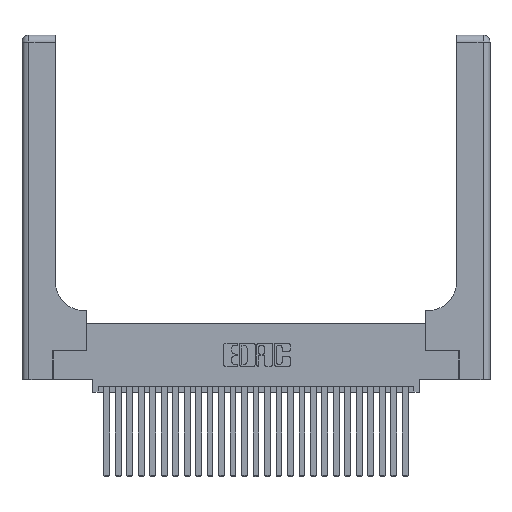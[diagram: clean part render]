
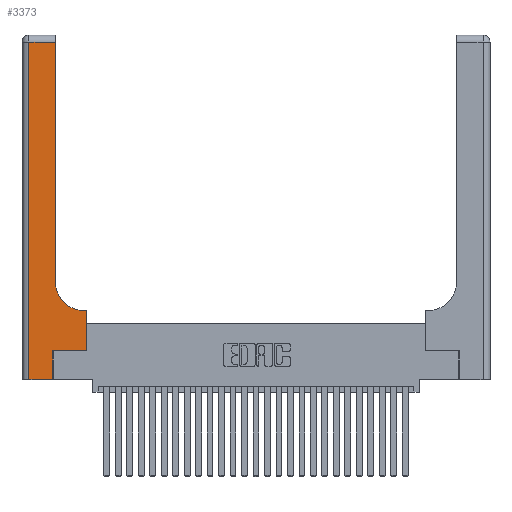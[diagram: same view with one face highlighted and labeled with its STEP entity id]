
A CAD part, top view. The second image highlights one B-rep face of the part: STEP entity #3373.
In plain terms, the highlighted planar face has unit normal (0, 0, 1).
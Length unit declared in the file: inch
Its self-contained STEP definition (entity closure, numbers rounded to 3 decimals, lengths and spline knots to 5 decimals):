
#2364 = CARTESIAN_POINT ( 'NONE',  ( 0.269, 0., 0.37 ) ) ;
#2859 = CARTESIAN_POINT ( 'NONE',  ( 0.2915, 3., 0.37 ) ) ;
#2923 = CARTESIAN_POINT ( 'NONE',  ( 0.2915, 2.94, 0.37 ) ) ;
#2935 = EDGE_CURVE ( 'NONE', #10302, #12934, #21000, .T. ) ;
#3134 = LINE ( 'NONE', #16688, #11346 ) ;
#3373 = ADVANCED_FACE ( 'NONE', ( #4722 ), #11329, .F. ) ;
#3990 = CARTESIAN_POINT ( 'NONE',  ( 0.269, 0.25, 0.37 ) ) ;
#4154 = ORIENTED_EDGE ( 'NONE', *, *, #14127, .T. ) ;
#4536 = DIRECTION ( 'NONE',  ( 0., 1., 0. ) ) ;
#4601 = ORIENTED_EDGE ( 'NONE', *, *, #17300, .T. ) ;
#4671 = CARTESIAN_POINT ( 'NONE',  ( 0.06, 3., 0.37 ) ) ;
#4722 = FACE_OUTER_BOUND ( 'NONE', #21635, .T. ) ;
#4834 = CARTESIAN_POINT ( 'NONE',  ( 0.269, 0.25, 0.37 ) ) ;
#4879 = CARTESIAN_POINT ( 'NONE',  ( 0., 3., 0.37 ) ) ;
#4957 = DIRECTION ( 'NONE',  ( 1., 0., 0. ) ) ;
#5031 = DIRECTION ( 'NONE',  ( 0., 1., 0. ) ) ;
#5175 = DIRECTION ( 'NONE',  ( 0., 1., 0. ) ) ;
#5514 = VECTOR ( 'NONE', #4957, 39.37008 ) ;
#5590 = VECTOR ( 'NONE', #5175, 39.37008 ) ;
#5608 = CIRCLE ( 'NONE', #23558, 0.25 ) ;
#6790 = DIRECTION ( 'NONE',  ( 0., -1., 0. ) ) ;
#6842 = CARTESIAN_POINT ( 'NONE',  ( 0.269, 0., 0.37 ) ) ;
#6924 = VERTEX_POINT ( 'NONE', #21004 ) ;
#7372 = CARTESIAN_POINT ( 'NONE',  ( 0.06, 2.94, 0.37 ) ) ;
#7584 = VERTEX_POINT ( 'NONE', #26493 ) ;
#8196 = VERTEX_POINT ( 'NONE', #23584 ) ;
#8444 = EDGE_CURVE ( 'NONE', #8196, #7584, #10663, .T. ) ;
#8859 = VECTOR ( 'NONE', #5031, 39.37008 ) ;
#8915 = ORIENTED_EDGE ( 'NONE', *, *, #8444, .T. ) ;
#9734 = EDGE_CURVE ( 'NONE', #12934, #21002, #12864, .T. ) ;
#10302 = VERTEX_POINT ( 'NONE', #7372 ) ;
#10546 = DIRECTION ( 'NONE',  ( -1., 0., 0. ) ) ;
#10648 = ORIENTED_EDGE ( 'NONE', *, *, #25148, .T. ) ;
#10663 = LINE ( 'NONE', #16433, #12419 ) ;
#11214 = VERTEX_POINT ( 'NONE', #3990 ) ;
#11329 = PLANE ( 'NONE',  #25306 ) ;
#11346 = VECTOR ( 'NONE', #10546, 39.37008 ) ;
#12419 = VECTOR ( 'NONE', #16619, 39.37008 ) ;
#12864 = LINE ( 'NONE', #22420, #5514 ) ;
#12934 = VERTEX_POINT ( 'NONE', #14301 ) ;
#14127 = EDGE_CURVE ( 'NONE', #6924, #8196, #26868, .T. ) ;
#14301 = CARTESIAN_POINT ( 'NONE',  ( 0.06, 0., 0.37 ) ) ;
#15295 = EDGE_CURVE ( 'NONE', #21002, #11214, #24083, .T. ) ;
#16262 = VERTEX_POINT ( 'NONE', #2923 ) ;
#16278 = VECTOR ( 'NONE', #20381, 39.37008 ) ;
#16433 = CARTESIAN_POINT ( 'NONE',  ( 0.2915, 0.6, 0.37 ) ) ;
#16619 = DIRECTION ( 'NONE',  ( -1., 0., 0. ) ) ;
#16688 = CARTESIAN_POINT ( 'NONE',  ( 0., 2.94, 0.37 ) ) ;
#16888 = CARTESIAN_POINT ( 'NONE',  ( 0.2915, 0.85, 0.37 ) ) ;
#17300 = EDGE_CURVE ( 'NONE', #21382, #16262, #20516, .T. ) ;
#19340 = LINE ( 'NONE', #4834, #16278 ) ;
#19821 = ORIENTED_EDGE ( 'NONE', *, *, #22510, .T. ) ;
#19901 = ORIENTED_EDGE ( 'NONE', *, *, #15295, .T. ) ;
#20381 = DIRECTION ( 'NONE',  ( 1., 0., 0. ) ) ;
#20422 = EDGE_CURVE ( 'NONE', #11214, #6924, #19340, .T. ) ;
#20483 = ORIENTED_EDGE ( 'NONE', *, *, #20422, .T. ) ;
#20516 = LINE ( 'NONE', #2859, #8859 ) ;
#20991 = VECTOR ( 'NONE', #4536, 39.37008 ) ;
#21000 = LINE ( 'NONE', #4671, #22032 ) ;
#21002 = VERTEX_POINT ( 'NONE', #2364 ) ;
#21004 = CARTESIAN_POINT ( 'NONE',  ( 0.5585, 0.25, 0.37 ) ) ;
#21382 = VERTEX_POINT ( 'NONE', #16888 ) ;
#21415 = ORIENTED_EDGE ( 'NONE', *, *, #9734, .T. ) ;
#21635 = EDGE_LOOP ( 'NONE', ( #4601, #19821, #27009, #21415, #19901, #20483, #4154, #8915, #10648 ) ) ;
#22032 = VECTOR ( 'NONE', #6790, 39.37008 ) ;
#22420 = CARTESIAN_POINT ( 'NONE',  ( 0., 0., 0.37 ) ) ;
#22437 = DIRECTION ( 'NONE',  ( -1., 0., 0. ) ) ;
#22510 = EDGE_CURVE ( 'NONE', #16262, #10302, #3134, .T. ) ;
#22622 = CARTESIAN_POINT ( 'NONE',  ( 0.5585, 0.25, 0.37 ) ) ;
#23558 = AXIS2_PLACEMENT_3D ( 'NONE', #25719, #27049, #25697 ) ;
#23584 = CARTESIAN_POINT ( 'NONE',  ( 0.5585, 0.6, 0.37 ) ) ;
#24083 = LINE ( 'NONE', #6842, #20991 ) ;
#25148 = EDGE_CURVE ( 'NONE', #7584, #21382, #5608, .T. ) ;
#25306 = AXIS2_PLACEMENT_3D ( 'NONE', #4879, #26759, #22437 ) ;
#25697 = DIRECTION ( 'NONE',  ( 1., 0., 0. ) ) ;
#25719 = CARTESIAN_POINT ( 'NONE',  ( 0.5415, 0.85, 0.37 ) ) ;
#26493 = CARTESIAN_POINT ( 'NONE',  ( 0.5415, 0.6, 0.37 ) ) ;
#26759 = DIRECTION ( 'NONE',  ( 0., 0., -1. ) ) ;
#26868 = LINE ( 'NONE', #22622, #5590 ) ;
#27009 = ORIENTED_EDGE ( 'NONE', *, *, #2935, .T. ) ;
#27049 = DIRECTION ( 'NONE',  ( 0., 0., -1. ) ) ;
